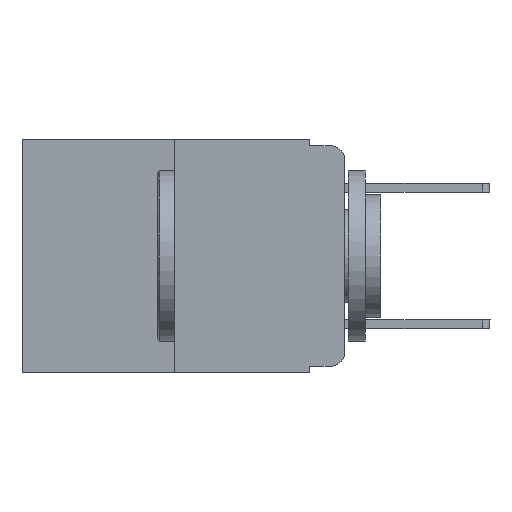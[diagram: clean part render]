
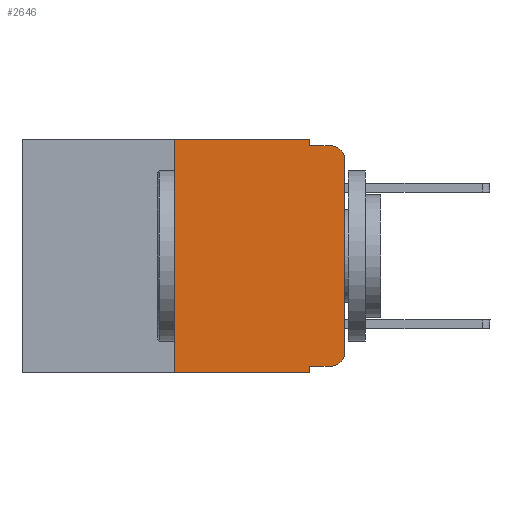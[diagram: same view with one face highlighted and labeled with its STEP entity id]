
A CAD part, left-side view. The second image highlights one B-rep face of the part: STEP entity #2646.
In plain terms, the highlighted planar face has unit normal (-1, 0, 0).
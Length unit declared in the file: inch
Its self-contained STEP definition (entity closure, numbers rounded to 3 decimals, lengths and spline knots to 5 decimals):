
#943 = AXIS2_PLACEMENT_3D ( 'NONE', #9018, #15484, #5419 ) ;
#1223 = CIRCLE ( 'NONE', #943, 0.02 ) ;
#1321 = ORIENTED_EDGE ( 'NONE', *, *, #6558, .F. ) ;
#1650 = AXIS2_PLACEMENT_3D ( 'NONE', #6659, #15412, #8090 ) ;
#1755 = DIRECTION ( 'NONE',  ( 0., -1., 0. ) ) ;
#1813 = VERTEX_POINT ( 'NONE', #8737 ) ;
#1973 = CARTESIAN_POINT ( 'NONE',  ( 0., 0.25, 0. ) ) ;
#2257 = DIRECTION ( 'NONE',  ( 0., -1., 0. ) ) ;
#2344 = VECTOR ( 'NONE', #4650, 39.37008 ) ;
#2646 = ADVANCED_FACE ( 'NONE', ( #11924 ), #14097, .F. ) ;
#2769 = LINE ( 'NONE', #4413, #6310 ) ;
#2910 = VERTEX_POINT ( 'NONE', #16050 ) ;
#2983 = ORIENTED_EDGE ( 'NONE', *, *, #7840, .F. ) ;
#3151 = LINE ( 'NONE', #14618, #2344 ) ;
#3153 = VERTEX_POINT ( 'NONE', #10149 ) ;
#3232 = EDGE_CURVE ( 'NONE', #2910, #3153, #9288, .T. ) ;
#3372 = LINE ( 'NONE', #14790, #15505 ) ;
#3430 = CARTESIAN_POINT ( 'NONE',  ( 0., 0.051, -0.01 ) ) ;
#3818 = ORIENTED_EDGE ( 'NONE', *, *, #14319, .T. ) ;
#3824 = VECTOR ( 'NONE', #10025, 39.37008 ) ;
#3956 = CARTESIAN_POINT ( 'NONE',  ( 0., 0., 0. ) ) ;
#3990 = ORIENTED_EDGE ( 'NONE', *, *, #13067, .T. ) ;
#4163 = ORIENTED_EDGE ( 'NONE', *, *, #11758, .F. ) ;
#4352 = DIRECTION ( 'NONE',  ( 0., -1., 0. ) ) ;
#4363 = VECTOR ( 'NONE', #9575, 39.37008 ) ;
#4413 = CARTESIAN_POINT ( 'NONE',  ( 0., 0.051, 0. ) ) ;
#4650 = DIRECTION ( 'NONE',  ( 0., 0., 1. ) ) ;
#4804 = VERTEX_POINT ( 'NONE', #7699 ) ;
#4853 = CARTESIAN_POINT ( 'NONE',  ( 0., 0.051, -0.343 ) ) ;
#5014 = ORIENTED_EDGE ( 'NONE', *, *, #11794, .F. ) ;
#5419 = DIRECTION ( 'NONE',  ( 0., 0., -1. ) ) ;
#5525 = VECTOR ( 'NONE', #1755, 39.37008 ) ;
#5935 = EDGE_CURVE ( 'NONE', #12492, #2910, #11681, .T. ) ;
#6310 = VECTOR ( 'NONE', #10180, 39.37008 ) ;
#6558 = EDGE_CURVE ( 'NONE', #13899, #3153, #8463, .T. ) ;
#6659 = CARTESIAN_POINT ( 'NONE',  ( 0., 0.473, 0. ) ) ;
#6788 = CARTESIAN_POINT ( 'NONE',  ( 0., 0.051, -0.333 ) ) ;
#6790 = AXIS2_PLACEMENT_3D ( 'NONE', #10563, #8073, #9211 ) ;
#6839 = EDGE_CURVE ( 'NONE', #8345, #12720, #2769, .T. ) ;
#7421 = LINE ( 'NONE', #10603, #15459 ) ;
#7699 = CARTESIAN_POINT ( 'NONE',  ( 0., 0.25, -0.343 ) ) ;
#7840 = EDGE_CURVE ( 'NONE', #4804, #13276, #3151, .T. ) ;
#8073 = DIRECTION ( 'NONE',  ( -1., 0., 0. ) ) ;
#8090 = DIRECTION ( 'NONE',  ( 0., 0., -1. ) ) ;
#8345 = VERTEX_POINT ( 'NONE', #6788 ) ;
#8463 = LINE ( 'NONE', #11233, #15712 ) ;
#8737 = CARTESIAN_POINT ( 'NONE',  ( 0., 0.051, 0. ) ) ;
#8835 = ORIENTED_EDGE ( 'NONE', *, *, #6839, .F. ) ;
#9018 = CARTESIAN_POINT ( 'NONE',  ( 0., 0.02, -0.313 ) ) ;
#9211 = DIRECTION ( 'NONE',  ( 0., 0., -1. ) ) ;
#9235 = LINE ( 'NONE', #15977, #4363 ) ;
#9288 = CIRCLE ( 'NONE', #6790, 0.02 ) ;
#9354 = ORIENTED_EDGE ( 'NONE', *, *, #5935, .T. ) ;
#9575 = DIRECTION ( 'NONE',  ( 0., 0., -1. ) ) ;
#9898 = CARTESIAN_POINT ( 'NONE',  ( 0., 0., -0.313 ) ) ;
#10025 = DIRECTION ( 'NONE',  ( 0., 0., 1. ) ) ;
#10149 = CARTESIAN_POINT ( 'NONE',  ( 0., 0.02, -0.01 ) ) ;
#10180 = DIRECTION ( 'NONE',  ( 0., 0., -1. ) ) ;
#10563 = CARTESIAN_POINT ( 'NONE',  ( 0., 0.02, -0.03 ) ) ;
#10603 = CARTESIAN_POINT ( 'NONE',  ( 0., 0.051, -0.333 ) ) ;
#11233 = CARTESIAN_POINT ( 'NONE',  ( 0., 0.051, -0.01 ) ) ;
#11415 = LINE ( 'NONE', #15254, #5525 ) ;
#11681 = LINE ( 'NONE', #3956, #3824 ) ;
#11758 = EDGE_CURVE ( 'NONE', #13276, #1813, #3372, .T. ) ;
#11794 = EDGE_CURVE ( 'NONE', #1813, #13899, #9235, .T. ) ;
#11924 = FACE_OUTER_BOUND ( 'NONE', #14533, .T. ) ;
#12492 = VERTEX_POINT ( 'NONE', #9898 ) ;
#12720 = VERTEX_POINT ( 'NONE', #4853 ) ;
#13056 = EDGE_CURVE ( 'NONE', #14451, #12492, #1223, .T. ) ;
#13067 = EDGE_CURVE ( 'NONE', #4804, #12720, #11415, .T. ) ;
#13276 = VERTEX_POINT ( 'NONE', #1973 ) ;
#13608 = DIRECTION ( 'NONE',  ( 0., -1., 0. ) ) ;
#13899 = VERTEX_POINT ( 'NONE', #3430 ) ;
#14097 = PLANE ( 'NONE',  #1650 ) ;
#14319 = EDGE_CURVE ( 'NONE', #8345, #14451, #7421, .T. ) ;
#14451 = VERTEX_POINT ( 'NONE', #15704 ) ;
#14533 = EDGE_LOOP ( 'NONE', ( #9354, #14597, #1321, #5014, #4163, #2983, #3990, #8835, #3818, #15456 ) ) ;
#14597 = ORIENTED_EDGE ( 'NONE', *, *, #3232, .T. ) ;
#14618 = CARTESIAN_POINT ( 'NONE',  ( 0., 0.25, 0. ) ) ;
#14790 = CARTESIAN_POINT ( 'NONE',  ( 0., 0.473, 0. ) ) ;
#15254 = CARTESIAN_POINT ( 'NONE',  ( 0., 0.473, -0.343 ) ) ;
#15412 = DIRECTION ( 'NONE',  ( 1., 0., 0. ) ) ;
#15456 = ORIENTED_EDGE ( 'NONE', *, *, #13056, .T. ) ;
#15459 = VECTOR ( 'NONE', #4352, 39.37008 ) ;
#15484 = DIRECTION ( 'NONE',  ( -1., 0., 0. ) ) ;
#15505 = VECTOR ( 'NONE', #2257, 39.37008 ) ;
#15704 = CARTESIAN_POINT ( 'NONE',  ( 0., 0.02, -0.333 ) ) ;
#15712 = VECTOR ( 'NONE', #13608, 39.37008 ) ;
#15977 = CARTESIAN_POINT ( 'NONE',  ( 0., 0.051, 0. ) ) ;
#16050 = CARTESIAN_POINT ( 'NONE',  ( 0., 0., -0.03 ) ) ;
